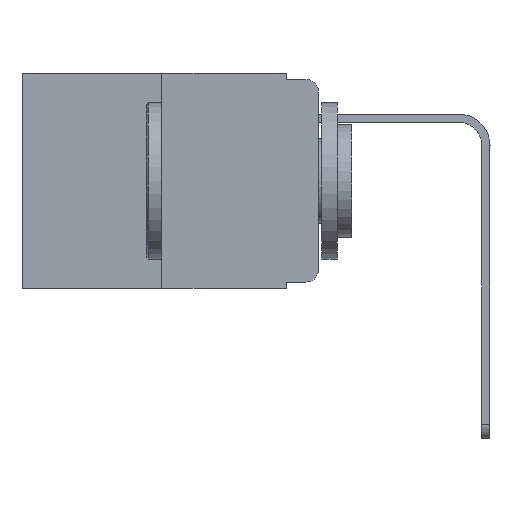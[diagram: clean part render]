
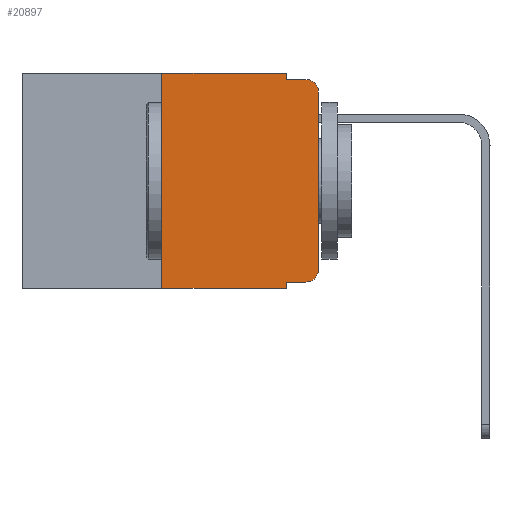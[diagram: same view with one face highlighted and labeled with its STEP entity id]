
A CAD part, left-side view. The second image highlights one B-rep face of the part: STEP entity #20897.
In plain terms, the highlighted planar face has unit normal (-1, 0, 0).
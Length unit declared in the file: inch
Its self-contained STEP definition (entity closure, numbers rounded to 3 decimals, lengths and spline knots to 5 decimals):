
#393 = DIRECTION ( 'NONE',  ( 0., -1., 0. ) ) ;
#567 = AXIS2_PLACEMENT_3D ( 'NONE', #17818, #21748, #4741 ) ;
#1423 = DIRECTION ( 'NONE',  ( 0., 0., -1. ) ) ;
#2443 = VERTEX_POINT ( 'NONE', #17422 ) ;
#2827 = ORIENTED_EDGE ( 'NONE', *, *, #9446, .T. ) ;
#3046 = LINE ( 'NONE', #18097, #9617 ) ;
#3707 = CARTESIAN_POINT ( 'NONE',  ( 0., 0.02, -0.03 ) ) ;
#3890 = VECTOR ( 'NONE', #24345, 39.37008 ) ;
#3962 = CARTESIAN_POINT ( 'NONE',  ( 0., 0.02, -0.01 ) ) ;
#4219 = VERTEX_POINT ( 'NONE', #23066 ) ;
#4738 = ORIENTED_EDGE ( 'NONE', *, *, #4751, .F. ) ;
#4741 = DIRECTION ( 'NONE',  ( 0., 0., -1. ) ) ;
#4751 = EDGE_CURVE ( 'NONE', #4219, #13989, #5879, .T. ) ;
#4952 = AXIS2_PLACEMENT_3D ( 'NONE', #5201, #12885, #1423 ) ;
#5061 = ORIENTED_EDGE ( 'NONE', *, *, #8056, .T. ) ;
#5201 = CARTESIAN_POINT ( 'NONE',  ( 0., 0.473, 0. ) ) ;
#5593 = VERTEX_POINT ( 'NONE', #3962 ) ;
#5625 = EDGE_CURVE ( 'NONE', #2443, #18699, #7228, .T. ) ;
#5849 = EDGE_CURVE ( 'NONE', #19479, #4219, #3046, .T. ) ;
#5879 = LINE ( 'NONE', #13684, #17490 ) ;
#5889 = CARTESIAN_POINT ( 'NONE',  ( 0., 0.473, -0.343 ) ) ;
#6349 = EDGE_LOOP ( 'NONE', ( #14350, #8538, #22271, #4738, #15547, #6746, #5061, #18189, #13189, #2827 ) ) ;
#6746 = ORIENTED_EDGE ( 'NONE', *, *, #19003, .F. ) ;
#7228 = LINE ( 'NONE', #17025, #21833 ) ;
#7448 = VECTOR ( 'NONE', #13639, 39.37008 ) ;
#7633 = DIRECTION ( 'NONE',  ( -1., 0., 0. ) ) ;
#7982 = CIRCLE ( 'NONE', #567, 0.02 ) ;
#8056 = EDGE_CURVE ( 'NONE', #9199, #14192, #13716, .T. ) ;
#8279 = DIRECTION ( 'NONE',  ( 0., 0., 1. ) ) ;
#8427 = EDGE_CURVE ( 'NONE', #13989, #5593, #20524, .T. ) ;
#8481 = FACE_OUTER_BOUND ( 'NONE', #6349, .T. ) ;
#8530 = CARTESIAN_POINT ( 'NONE',  ( 0., 0.051, -0.01 ) ) ;
#8538 = ORIENTED_EDGE ( 'NONE', *, *, #12876, .T. ) ;
#8995 = CARTESIAN_POINT ( 'NONE',  ( 0., 0., -0.03 ) ) ;
#9110 = VERTEX_POINT ( 'NONE', #24478 ) ;
#9199 = VERTEX_POINT ( 'NONE', #13346 ) ;
#9446 = EDGE_CURVE ( 'NONE', #9110, #2443, #7982, .T. ) ;
#9617 = VECTOR ( 'NONE', #23685, 39.37008 ) ;
#9899 = AXIS2_PLACEMENT_3D ( 'NONE', #3707, #7633, #20947 ) ;
#10701 = VECTOR ( 'NONE', #393, 39.37008 ) ;
#11559 = DIRECTION ( 'NONE',  ( 0., -1., 0. ) ) ;
#12876 = EDGE_CURVE ( 'NONE', #18699, #5593, #15345, .T. ) ;
#12885 = DIRECTION ( 'NONE',  ( 1., 0., 0. ) ) ;
#13143 = CARTESIAN_POINT ( 'NONE',  ( 0., 0.051, -0.01 ) ) ;
#13189 = ORIENTED_EDGE ( 'NONE', *, *, #17732, .T. ) ;
#13346 = CARTESIAN_POINT ( 'NONE',  ( 0., 0.25, -0.343 ) ) ;
#13639 = DIRECTION ( 'NONE',  ( 0., -1., 0. ) ) ;
#13684 = CARTESIAN_POINT ( 'NONE',  ( 0., 0.051, 0. ) ) ;
#13706 = LINE ( 'NONE', #21236, #10701 ) ;
#13716 = LINE ( 'NONE', #5889, #7448 ) ;
#13989 = VERTEX_POINT ( 'NONE', #8530 ) ;
#14192 = VERTEX_POINT ( 'NONE', #24372 ) ;
#14350 = ORIENTED_EDGE ( 'NONE', *, *, #5625, .T. ) ;
#15159 = CARTESIAN_POINT ( 'NONE',  ( 0., 0.051, -0.333 ) ) ;
#15345 = CIRCLE ( 'NONE', #9899, 0.02 ) ;
#15488 = VECTOR ( 'NONE', #11559, 39.37008 ) ;
#15547 = ORIENTED_EDGE ( 'NONE', *, *, #5849, .F. ) ;
#16084 = CARTESIAN_POINT ( 'NONE',  ( 0., 0.25, 0. ) ) ;
#16584 = CARTESIAN_POINT ( 'NONE',  ( 0., 0.25, 0. ) ) ;
#16604 = PLANE ( 'NONE',  #4952 ) ;
#16971 = LINE ( 'NONE', #20678, #3890 ) ;
#17025 = CARTESIAN_POINT ( 'NONE',  ( 0., 0., 0. ) ) ;
#17422 = CARTESIAN_POINT ( 'NONE',  ( 0., 0., -0.313 ) ) ;
#17490 = VECTOR ( 'NONE', #19344, 39.37008 ) ;
#17494 = LINE ( 'NONE', #16084, #21964 ) ;
#17732 = EDGE_CURVE ( 'NONE', #21539, #9110, #13706, .T. ) ;
#17818 = CARTESIAN_POINT ( 'NONE',  ( 0., 0.02, -0.313 ) ) ;
#18097 = CARTESIAN_POINT ( 'NONE',  ( 0., 0.473, 0. ) ) ;
#18189 = ORIENTED_EDGE ( 'NONE', *, *, #23815, .F. ) ;
#18699 = VERTEX_POINT ( 'NONE', #8995 ) ;
#19003 = EDGE_CURVE ( 'NONE', #9199, #19479, #17494, .T. ) ;
#19344 = DIRECTION ( 'NONE',  ( 0., 0., -1. ) ) ;
#19479 = VERTEX_POINT ( 'NONE', #16584 ) ;
#20524 = LINE ( 'NONE', #13143, #15488 ) ;
#20678 = CARTESIAN_POINT ( 'NONE',  ( 0., 0.051, 0. ) ) ;
#20897 = ADVANCED_FACE ( 'NONE', ( #8481 ), #16604, .F. ) ;
#20947 = DIRECTION ( 'NONE',  ( 0., 0., -1. ) ) ;
#21236 = CARTESIAN_POINT ( 'NONE',  ( 0., 0.051, -0.333 ) ) ;
#21539 = VERTEX_POINT ( 'NONE', #15159 ) ;
#21748 = DIRECTION ( 'NONE',  ( -1., 0., 0. ) ) ;
#21833 = VECTOR ( 'NONE', #23039, 39.37008 ) ;
#21964 = VECTOR ( 'NONE', #8279, 39.37008 ) ;
#22271 = ORIENTED_EDGE ( 'NONE', *, *, #8427, .F. ) ;
#23039 = DIRECTION ( 'NONE',  ( 0., 0., 1. ) ) ;
#23066 = CARTESIAN_POINT ( 'NONE',  ( 0., 0.051, 0. ) ) ;
#23685 = DIRECTION ( 'NONE',  ( 0., -1., 0. ) ) ;
#23815 = EDGE_CURVE ( 'NONE', #21539, #14192, #16971, .T. ) ;
#24345 = DIRECTION ( 'NONE',  ( 0., 0., -1. ) ) ;
#24372 = CARTESIAN_POINT ( 'NONE',  ( 0., 0.051, -0.343 ) ) ;
#24478 = CARTESIAN_POINT ( 'NONE',  ( 0., 0.02, -0.333 ) ) ;
